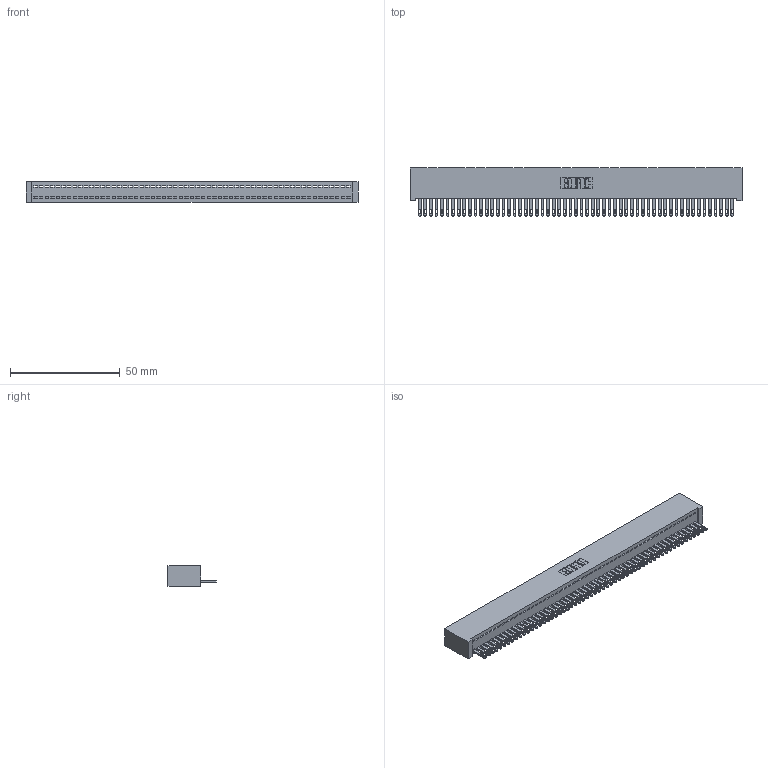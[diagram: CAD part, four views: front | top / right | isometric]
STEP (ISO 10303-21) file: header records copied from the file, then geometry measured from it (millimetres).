
FILE_DESCRIPTION (( 'STEP AP203' ), '1' );
FILE_NAME ('892-057-500-101.STEP', '2020-09-21T18:48:17', ( '' ), ( '' ), 'SwSTEP 2.0', 'SolidWorks 2020', '' );
FILE_SCHEMA (( 'CONFIG_CONTROL_DESIGN' ));
Length unit declared in the file: inch
Products named in the file (3): 892-057-500-101; 842 Part_Lugless; 345-292-001_345-293-100
Assembly tree (58 placements, depth 2):
  892-057-500-101
    842 Part_Lugless
    345-292-001_345-293-100  x57
Bounding box: 151.03 x 21.85 x 9.4 mm (x, y, z)
Volume: 13741.7 mm3; surface area: 20894.6 mm2
Topology: 58 solids, 58 shells, 3180 faces, 9851 edges, 6566 vertices
Faces by surface type: plane 2114, cylinder 1066
Entity records: 32427 total; most frequent: CARTESIAN_POINT 5597, ORIENTED_EDGE 5590, DIRECTION 4685, EDGE_CURVE 2795, LINE 2671, VECTOR 2671, VERTEX_POINT 1862, AXIS2_PLACEMENT_3D 1007
